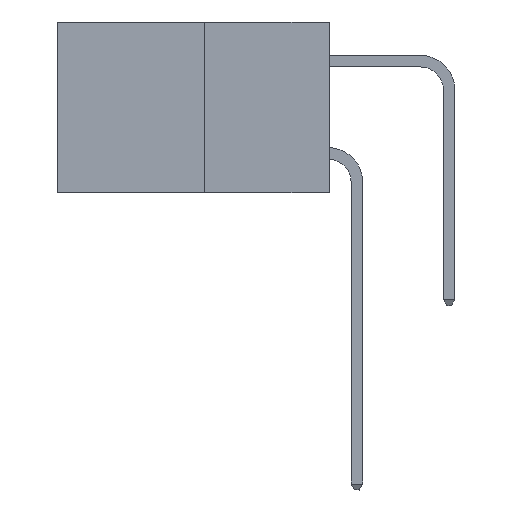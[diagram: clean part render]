
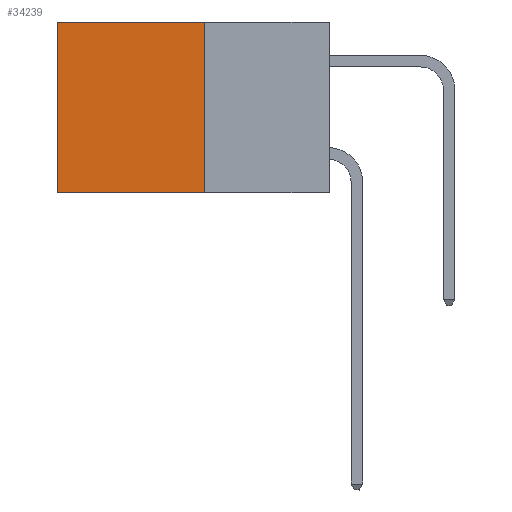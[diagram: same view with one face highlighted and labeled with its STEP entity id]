
A CAD part, left-side view. The second image highlights one B-rep face of the part: STEP entity #34239.
In plain terms, the highlighted planar face has unit normal (-1, 0, 0).
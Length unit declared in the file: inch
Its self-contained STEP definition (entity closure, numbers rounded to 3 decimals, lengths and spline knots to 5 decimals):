
#729 = EDGE_CURVE ( 'NONE', #6619, #16707, #16059, .T. ) ;
#1828 = CARTESIAN_POINT ( 'NONE',  ( 0.277, 0.27, 0. ) ) ;
#3644 = VERTEX_POINT ( 'NONE', #27253 ) ;
#4538 = VECTOR ( 'NONE', #34862, 39.37008 ) ;
#5944 = VERTEX_POINT ( 'NONE', #1828 ) ;
#6619 = VERTEX_POINT ( 'NONE', #25048 ) ;
#6732 = VECTOR ( 'NONE', #36219, 39.37008 ) ;
#8085 = DIRECTION ( 'NONE',  ( 0., 1., 0. ) ) ;
#9130 = EDGE_LOOP ( 'NONE', ( #19236, #34482, #37443, #15738 ) ) ;
#14508 = EDGE_CURVE ( 'NONE', #3644, #16707, #37111, .T. ) ;
#14610 = CARTESIAN_POINT ( 'NONE',  ( 0.277, 0.59, -0.37 ) ) ;
#15738 = ORIENTED_EDGE ( 'NONE', *, *, #29067, .T. ) ;
#16059 = LINE ( 'NONE', #30800, #21956 ) ;
#16707 = VERTEX_POINT ( 'NONE', #14610 ) ;
#17016 = CARTESIAN_POINT ( 'NONE',  ( 0.277, 0.27, -0.37 ) ) ;
#18849 = CARTESIAN_POINT ( 'NONE',  ( 0.277, 0.27, 0. ) ) ;
#19236 = ORIENTED_EDGE ( 'NONE', *, *, #729, .T. ) ;
#19519 = LINE ( 'NONE', #18849, #6732 ) ;
#19915 = DIRECTION ( 'NONE',  ( 0., 0., -1. ) ) ;
#21956 = VECTOR ( 'NONE', #30752, 39.37008 ) ;
#23618 = AXIS2_PLACEMENT_3D ( 'NONE', #17016, #37229, #19915 ) ;
#24690 = FACE_OUTER_BOUND ( 'NONE', #9130, .T. ) ;
#25048 = CARTESIAN_POINT ( 'NONE',  ( 0.277, 0.59, 0. ) ) ;
#25594 = CARTESIAN_POINT ( 'NONE',  ( 0.277, 0.27, -0.37 ) ) ;
#26197 = CARTESIAN_POINT ( 'NONE',  ( 0.277, 0.27, -0.37 ) ) ;
#27253 = CARTESIAN_POINT ( 'NONE',  ( 0.277, 0.27, -0.37 ) ) ;
#29067 = EDGE_CURVE ( 'NONE', #5944, #6619, #19519, .T. ) ;
#30381 = VECTOR ( 'NONE', #8085, 39.37008 ) ;
#30752 = DIRECTION ( 'NONE',  ( 0., 0., -1. ) ) ;
#30800 = CARTESIAN_POINT ( 'NONE',  ( 0.277, 0.59, -0.37 ) ) ;
#31493 = PLANE ( 'NONE',  #23618 ) ;
#34239 = ADVANCED_FACE ( 'NONE', ( #24690 ), #31493, .F. ) ;
#34351 = EDGE_CURVE ( 'NONE', #5944, #3644, #35501, .T. ) ;
#34482 = ORIENTED_EDGE ( 'NONE', *, *, #14508, .F. ) ;
#34862 = DIRECTION ( 'NONE',  ( 0., 0., -1. ) ) ;
#35501 = LINE ( 'NONE', #26197, #4538 ) ;
#36219 = DIRECTION ( 'NONE',  ( 0., 1., 0. ) ) ;
#37111 = LINE ( 'NONE', #25594, #30381 ) ;
#37229 = DIRECTION ( 'NONE',  ( 1., 0., 0. ) ) ;
#37443 = ORIENTED_EDGE ( 'NONE', *, *, #34351, .F. ) ;
